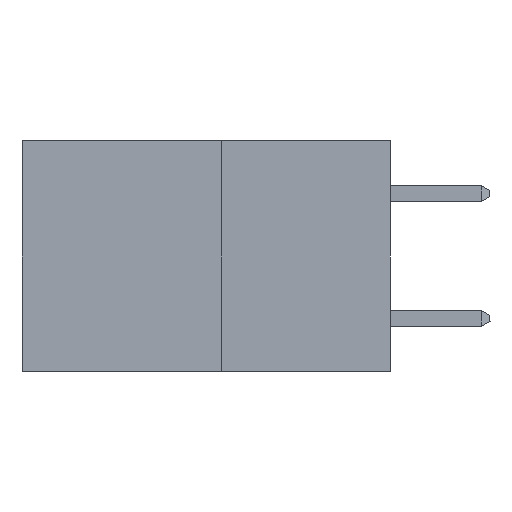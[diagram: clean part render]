
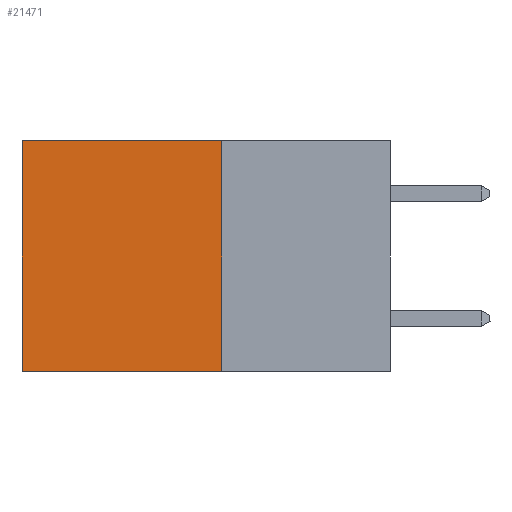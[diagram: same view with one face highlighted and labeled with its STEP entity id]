
A CAD part, left-side view. The second image highlights one B-rep face of the part: STEP entity #21471.
In plain terms, the highlighted planar face has unit normal (-1, 0, 0).
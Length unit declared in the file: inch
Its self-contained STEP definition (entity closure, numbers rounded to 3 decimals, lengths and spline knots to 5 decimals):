
#9 = CARTESIAN_POINT ( 'NONE',  ( 0.277, 0.27, -0.37 ) ) ;
#1579 = ORIENTED_EDGE ( 'NONE', *, *, #28374, .T. ) ;
#1708 = EDGE_CURVE ( 'NONE', #6008, #4492, #2136, .T. ) ;
#2136 = LINE ( 'NONE', #8354, #19737 ) ;
#2581 = DIRECTION ( 'NONE',  ( 1., 0., 0. ) ) ;
#3341 = CARTESIAN_POINT ( 'NONE',  ( 0.277, 0.59, -0.37 ) ) ;
#3788 = CARTESIAN_POINT ( 'NONE',  ( 0.277, 0.59, 0. ) ) ;
#4195 = LINE ( 'NONE', #21045, #26949 ) ;
#4492 = VERTEX_POINT ( 'NONE', #3341 ) ;
#5056 = VECTOR ( 'NONE', #9516, 39.37008 ) ;
#6008 = VERTEX_POINT ( 'NONE', #10490 ) ;
#6079 = EDGE_CURVE ( 'NONE', #22686, #11172, #18154, .T. ) ;
#8354 = CARTESIAN_POINT ( 'NONE',  ( 0.277, 0.27, -0.37 ) ) ;
#8658 = ORIENTED_EDGE ( 'NONE', *, *, #6079, .T. ) ;
#9516 = DIRECTION ( 'NONE',  ( 0., 1., 0. ) ) ;
#9657 = CARTESIAN_POINT ( 'NONE',  ( 0.277, 0.27, 0. ) ) ;
#10073 = DIRECTION ( 'NONE',  ( 0., 0., -1. ) ) ;
#10490 = CARTESIAN_POINT ( 'NONE',  ( 0.277, 0.27, -0.37 ) ) ;
#11172 = VERTEX_POINT ( 'NONE', #3788 ) ;
#11476 = FACE_OUTER_BOUND ( 'NONE', #25961, .T. ) ;
#12659 = DIRECTION ( 'NONE',  ( 0., 1., 0. ) ) ;
#13282 = ORIENTED_EDGE ( 'NONE', *, *, #24111, .F. ) ;
#15796 = CARTESIAN_POINT ( 'NONE',  ( 0.277, 0.27, -0.37 ) ) ;
#17711 = DIRECTION ( 'NONE',  ( 0., 0., -1. ) ) ;
#18021 = DIRECTION ( 'NONE',  ( 0., 0., -1. ) ) ;
#18154 = LINE ( 'NONE', #9657, #5056 ) ;
#19737 = VECTOR ( 'NONE', #12659, 39.37008 ) ;
#21045 = CARTESIAN_POINT ( 'NONE',  ( 0.277, 0.59, -0.37 ) ) ;
#21471 = ADVANCED_FACE ( 'NONE', ( #11476 ), #26815, .F. ) ;
#22686 = VERTEX_POINT ( 'NONE', #28493 ) ;
#24111 = EDGE_CURVE ( 'NONE', #22686, #6008, #24497, .T. ) ;
#24497 = LINE ( 'NONE', #9, #25186 ) ;
#25186 = VECTOR ( 'NONE', #17711, 39.37008 ) ;
#25961 = EDGE_LOOP ( 'NONE', ( #1579, #26479, #13282, #8658 ) ) ;
#26479 = ORIENTED_EDGE ( 'NONE', *, *, #1708, .F. ) ;
#26815 = PLANE ( 'NONE',  #27967 ) ;
#26949 = VECTOR ( 'NONE', #10073, 39.37008 ) ;
#27967 = AXIS2_PLACEMENT_3D ( 'NONE', #15796, #2581, #18021 ) ;
#28374 = EDGE_CURVE ( 'NONE', #11172, #4492, #4195, .T. ) ;
#28493 = CARTESIAN_POINT ( 'NONE',  ( 0.277, 0.27, 0. ) ) ;
